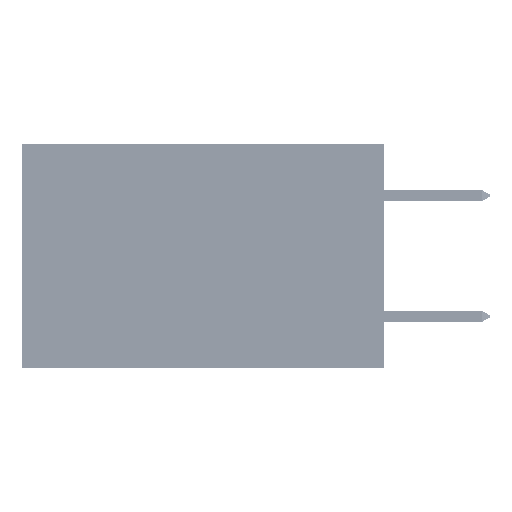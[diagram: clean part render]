
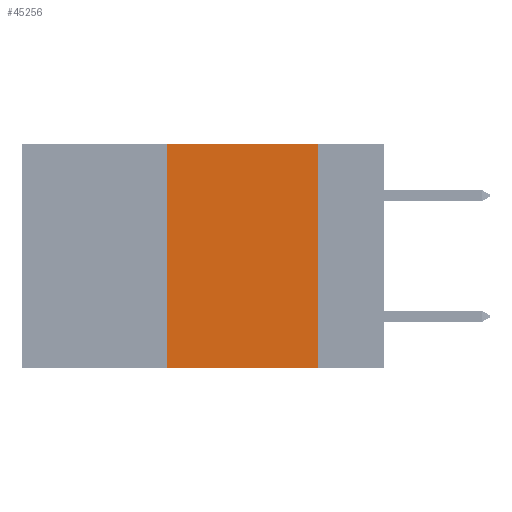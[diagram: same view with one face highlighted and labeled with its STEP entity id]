
A CAD part, left-side view. The second image highlights one B-rep face of the part: STEP entity #45256.
In plain terms, the highlighted planar face has unit normal (-1, 0, 0).
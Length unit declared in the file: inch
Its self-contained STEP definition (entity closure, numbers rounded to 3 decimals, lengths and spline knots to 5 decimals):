
#266 = ORIENTED_EDGE ( 'NONE', *, *, #13426, .F. ) ;
#3447 = ORIENTED_EDGE ( 'NONE', *, *, #34658, .F. ) ;
#3859 = EDGE_CURVE ( 'NONE', #17272, #15532, #13301, .T. ) ;
#4422 = VERTEX_POINT ( 'NONE', #36287 ) ;
#4576 = CARTESIAN_POINT ( 'NONE',  ( 0., 0.36, 0. ) ) ;
#4667 = DIRECTION ( 'NONE',  ( 0., 0., -1. ) ) ;
#7715 = AXIS2_PLACEMENT_3D ( 'NONE', #16262, #39563, #12319 ) ;
#12319 = DIRECTION ( 'NONE',  ( 0., 0., -1. ) ) ;
#12378 = VERTEX_POINT ( 'NONE', #49467 ) ;
#12514 = CARTESIAN_POINT ( 'NONE',  ( 0., 0.6, -0.37 ) ) ;
#12549 = CARTESIAN_POINT ( 'NONE',  ( 0., 0.11, 0. ) ) ;
#13301 = LINE ( 'NONE', #12514, #46472 ) ;
#13426 = EDGE_CURVE ( 'NONE', #12378, #4422, #44584, .T. ) ;
#13960 = EDGE_CURVE ( 'NONE', #4422, #15532, #28456, .T. ) ;
#14968 = ORIENTED_EDGE ( 'NONE', *, *, #13960, .F. ) ;
#15261 = ORIENTED_EDGE ( 'NONE', *, *, #3859, .T. ) ;
#15532 = VERTEX_POINT ( 'NONE', #34870 ) ;
#16262 = CARTESIAN_POINT ( 'NONE',  ( 0., 0.6, 0. ) ) ;
#17034 = DIRECTION ( 'NONE',  ( 0., -1., 0. ) ) ;
#17272 = VERTEX_POINT ( 'NONE', #25075 ) ;
#20643 = CARTESIAN_POINT ( 'NONE',  ( 0., 0.6, 0. ) ) ;
#20668 = DIRECTION ( 'NONE',  ( 0., 0., 1. ) ) ;
#23654 = DIRECTION ( 'NONE',  ( 0., -1., 0. ) ) ;
#25075 = CARTESIAN_POINT ( 'NONE',  ( 0., 0.36, -0.37 ) ) ;
#26506 = PLANE ( 'NONE',  #7715 ) ;
#28456 = LINE ( 'NONE', #12549, #45127 ) ;
#29545 = VECTOR ( 'NONE', #20668, 39.37008 ) ;
#33294 = EDGE_LOOP ( 'NONE', ( #14968, #266, #3447, #15261 ) ) ;
#34658 = EDGE_CURVE ( 'NONE', #17272, #12378, #35135, .T. ) ;
#34692 = FACE_OUTER_BOUND ( 'NONE', #33294, .T. ) ;
#34870 = CARTESIAN_POINT ( 'NONE',  ( 0., 0.11, -0.37 ) ) ;
#35135 = LINE ( 'NONE', #4576, #29545 ) ;
#36287 = CARTESIAN_POINT ( 'NONE',  ( 0., 0.11, 0. ) ) ;
#39563 = DIRECTION ( 'NONE',  ( 1., 0., 0. ) ) ;
#44584 = LINE ( 'NONE', #20643, #46411 ) ;
#45127 = VECTOR ( 'NONE', #4667, 39.37008 ) ;
#45256 = ADVANCED_FACE ( 'NONE', ( #34692 ), #26506, .F. ) ;
#46411 = VECTOR ( 'NONE', #17034, 39.37008 ) ;
#46472 = VECTOR ( 'NONE', #23654, 39.37008 ) ;
#49467 = CARTESIAN_POINT ( 'NONE',  ( 0., 0.36, 0. ) ) ;
